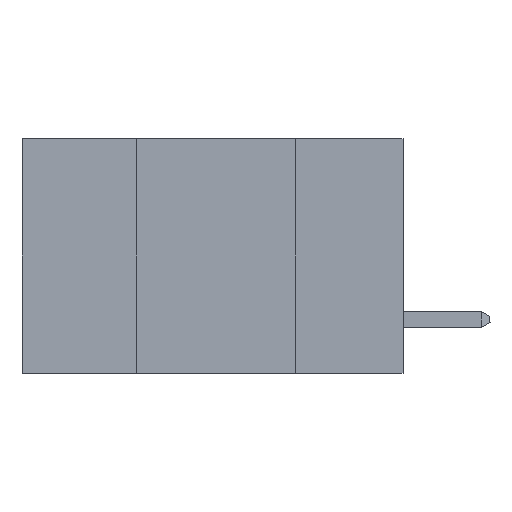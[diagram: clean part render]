
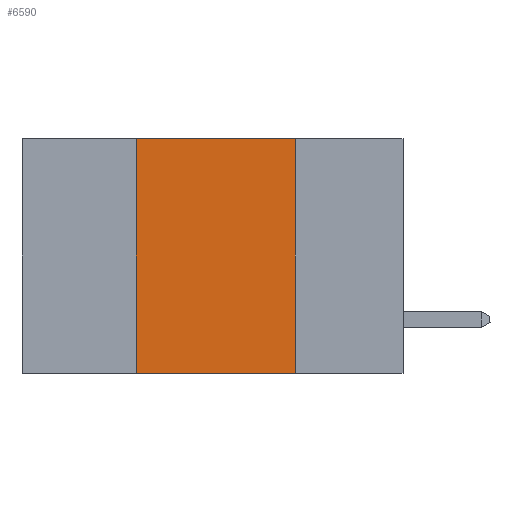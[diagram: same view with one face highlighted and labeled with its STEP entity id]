
A CAD part, left-side view. The second image highlights one B-rep face of the part: STEP entity #6590.
In plain terms, the highlighted planar face has unit normal (-1, 0, 0).
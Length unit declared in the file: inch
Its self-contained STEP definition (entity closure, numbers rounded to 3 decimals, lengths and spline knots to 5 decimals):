
#909 = VECTOR ( 'NONE', #25128, 39.37008 ) ;
#2929 = VECTOR ( 'NONE', #22896, 39.37008 ) ;
#3858 = LINE ( 'NONE', #38811, #2929 ) ;
#5482 = AXIS2_PLACEMENT_3D ( 'NONE', #12388, #27609, #24897 ) ;
#5491 = LINE ( 'NONE', #17709, #12177 ) ;
#5501 = EDGE_CURVE ( 'NONE', #10061, #8022, #5491, .T. ) ;
#6590 = ADVANCED_FACE ( 'NONE', ( #29876 ), #22105, .F. ) ;
#8022 = VERTEX_POINT ( 'NONE', #19365 ) ;
#9334 = EDGE_CURVE ( 'NONE', #29402, #10061, #11524, .T. ) ;
#10061 = VERTEX_POINT ( 'NONE', #26463 ) ;
#11364 = ORIENTED_EDGE ( 'NONE', *, *, #5501, .F. ) ;
#11524 = LINE ( 'NONE', #31150, #909 ) ;
#12177 = VECTOR ( 'NONE', #32793, 39.37008 ) ;
#12388 = CARTESIAN_POINT ( 'NONE',  ( 0., 0.6, 0. ) ) ;
#15024 = CARTESIAN_POINT ( 'NONE',  ( 0., 0.17, 0. ) ) ;
#17709 = CARTESIAN_POINT ( 'NONE',  ( 0., 0.6, 0. ) ) ;
#19365 = CARTESIAN_POINT ( 'NONE',  ( 0., 0.17, 0. ) ) ;
#19868 = EDGE_LOOP ( 'NONE', ( #29457, #11364, #38799, #22398 ) ) ;
#21894 = EDGE_CURVE ( 'NONE', #8022, #24807, #32508, .T. ) ;
#22105 = PLANE ( 'NONE',  #5482 ) ;
#22398 = ORIENTED_EDGE ( 'NONE', *, *, #26895, .T. ) ;
#22896 = DIRECTION ( 'NONE',  ( 0., -1., 0. ) ) ;
#24807 = VERTEX_POINT ( 'NONE', #30814 ) ;
#24897 = DIRECTION ( 'NONE',  ( 0., 0., -1. ) ) ;
#25128 = DIRECTION ( 'NONE',  ( 0., 0., 1. ) ) ;
#26463 = CARTESIAN_POINT ( 'NONE',  ( 0., 0.42, 0. ) ) ;
#26895 = EDGE_CURVE ( 'NONE', #29402, #24807, #3858, .T. ) ;
#27609 = DIRECTION ( 'NONE',  ( 1., 0., 0. ) ) ;
#29402 = VERTEX_POINT ( 'NONE', #33924 ) ;
#29457 = ORIENTED_EDGE ( 'NONE', *, *, #21894, .F. ) ;
#29876 = FACE_OUTER_BOUND ( 'NONE', #19868, .T. ) ;
#30814 = CARTESIAN_POINT ( 'NONE',  ( 0., 0.17, -0.37 ) ) ;
#31150 = CARTESIAN_POINT ( 'NONE',  ( 0., 0.42, 0. ) ) ;
#32508 = LINE ( 'NONE', #15024, #33465 ) ;
#32793 = DIRECTION ( 'NONE',  ( 0., -1., 0. ) ) ;
#33465 = VECTOR ( 'NONE', #36445, 39.37008 ) ;
#33924 = CARTESIAN_POINT ( 'NONE',  ( 0., 0.42, -0.37 ) ) ;
#36445 = DIRECTION ( 'NONE',  ( 0., 0., -1. ) ) ;
#38799 = ORIENTED_EDGE ( 'NONE', *, *, #9334, .F. ) ;
#38811 = CARTESIAN_POINT ( 'NONE',  ( 0., 0.6, -0.37 ) ) ;
